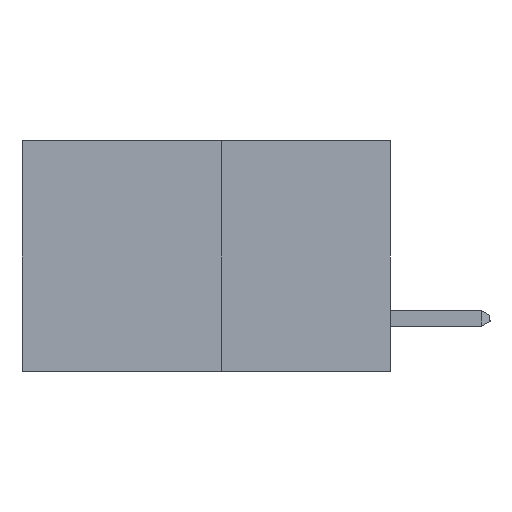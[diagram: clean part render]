
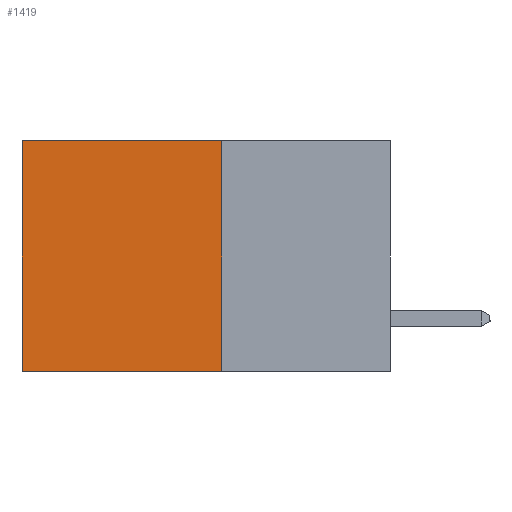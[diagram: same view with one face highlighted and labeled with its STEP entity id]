
A CAD part, left-side view. The second image highlights one B-rep face of the part: STEP entity #1419.
In plain terms, the highlighted planar face has unit normal (-1, 0, 0).
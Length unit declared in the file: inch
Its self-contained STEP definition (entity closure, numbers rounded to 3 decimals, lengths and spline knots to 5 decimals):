
#281 = VERTEX_POINT ( 'NONE', #7400 ) ;
#285 = DIRECTION ( 'NONE',  ( 0., 0., -1. ) ) ;
#682 = DIRECTION ( 'NONE',  ( 0., 1., 0. ) ) ;
#1419 = ADVANCED_FACE ( 'NONE', ( #7495 ), #3484, .F. ) ;
#1516 = LINE ( 'NONE', #7850, #7282 ) ;
#1530 = VECTOR ( 'NONE', #682, 39.37008 ) ;
#1684 = CARTESIAN_POINT ( 'NONE',  ( 0.277, 0.59, -0.37 ) ) ;
#2565 = LINE ( 'NONE', #11909, #13598 ) ;
#3484 = PLANE ( 'NONE',  #13607 ) ;
#3716 = VERTEX_POINT ( 'NONE', #11798 ) ;
#3776 = ORIENTED_EDGE ( 'NONE', *, *, #13127, .T. ) ;
#3808 = CARTESIAN_POINT ( 'NONE',  ( 0.277, 0.27, -0.37 ) ) ;
#4352 = LINE ( 'NONE', #1684, #7226 ) ;
#5641 = VERTEX_POINT ( 'NONE', #12814 ) ;
#5796 = DIRECTION ( 'NONE',  ( 0., 0., -1. ) ) ;
#7226 = VECTOR ( 'NONE', #9078, 39.37008 ) ;
#7282 = VECTOR ( 'NONE', #285, 39.37008 ) ;
#7400 = CARTESIAN_POINT ( 'NONE',  ( 0.277, 0.59, 0. ) ) ;
#7495 = FACE_OUTER_BOUND ( 'NONE', #13534, .T. ) ;
#7515 = EDGE_CURVE ( 'NONE', #13596, #3716, #2565, .T. ) ;
#7850 = CARTESIAN_POINT ( 'NONE',  ( 0.277, 0.27, -0.37 ) ) ;
#8193 = CARTESIAN_POINT ( 'NONE',  ( 0.277, 0.27, 0. ) ) ;
#8922 = CARTESIAN_POINT ( 'NONE',  ( 0.277, 0.27, -0.37 ) ) ;
#8953 = ORIENTED_EDGE ( 'NONE', *, *, #13517, .F. ) ;
#9078 = DIRECTION ( 'NONE',  ( 0., 0., -1. ) ) ;
#9553 = DIRECTION ( 'NONE',  ( 1., 0., 0. ) ) ;
#10450 = EDGE_CURVE ( 'NONE', #281, #3716, #4352, .T. ) ;
#11798 = CARTESIAN_POINT ( 'NONE',  ( 0.277, 0.59, -0.37 ) ) ;
#11851 = DIRECTION ( 'NONE',  ( 0., 1., 0. ) ) ;
#11855 = ORIENTED_EDGE ( 'NONE', *, *, #10450, .T. ) ;
#11909 = CARTESIAN_POINT ( 'NONE',  ( 0.277, 0.27, -0.37 ) ) ;
#12389 = LINE ( 'NONE', #8193, #1530 ) ;
#12814 = CARTESIAN_POINT ( 'NONE',  ( 0.277, 0.27, 0. ) ) ;
#12945 = ORIENTED_EDGE ( 'NONE', *, *, #7515, .F. ) ;
#13127 = EDGE_CURVE ( 'NONE', #5641, #281, #12389, .T. ) ;
#13517 = EDGE_CURVE ( 'NONE', #5641, #13596, #1516, .T. ) ;
#13534 = EDGE_LOOP ( 'NONE', ( #11855, #12945, #8953, #3776 ) ) ;
#13596 = VERTEX_POINT ( 'NONE', #8922 ) ;
#13598 = VECTOR ( 'NONE', #11851, 39.37008 ) ;
#13607 = AXIS2_PLACEMENT_3D ( 'NONE', #3808, #9553, #5796 ) ;
